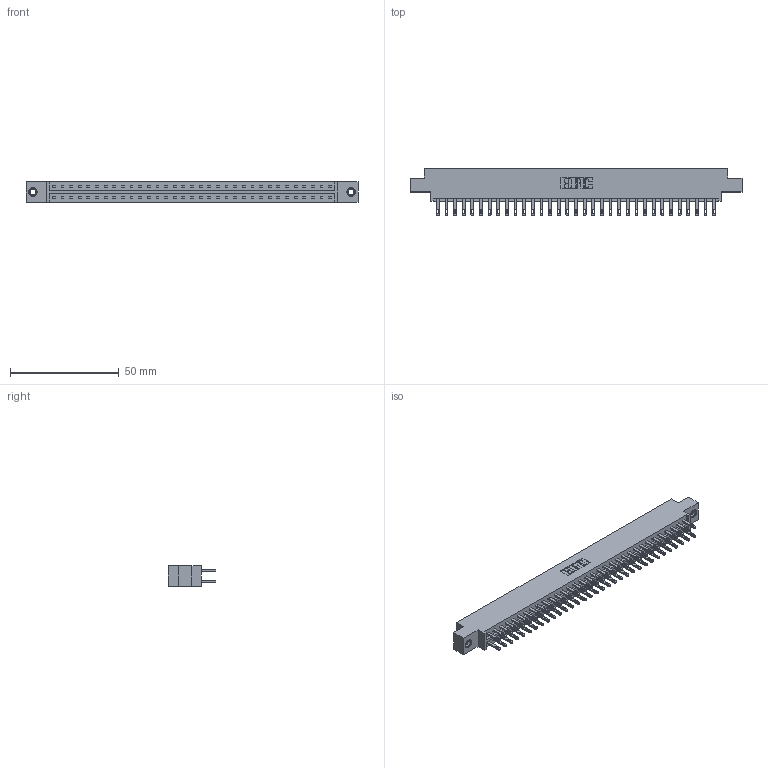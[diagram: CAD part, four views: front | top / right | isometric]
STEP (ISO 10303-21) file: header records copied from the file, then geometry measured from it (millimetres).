
FILE_DESCRIPTION (( 'STEP AP203' ), '1' );
FILE_NAME ('333-066-500-807.STEP', '2018-08-04T10:51:30', ( '' ), ( '' ), 'SwSTEP 2.0', 'SolidWorks 2016', '' );
FILE_SCHEMA (( 'CONFIG_CONTROL_DESIGN' ));
Length unit declared in the file: inch
Products named in the file (4): 333 Part_Offset - .156 Dia - TI; 345-292-001_345-293-100; 345-250-001_345-250-005-103; 333-066-500-807
Assembly tree (69 placements, depth 2):
  333-066-500-807
    333 Part_Offset - .156 Dia - TI
    345-292-001_345-293-100  x66
    345-250-001_345-250-005-103  x2
Bounding box: 152.3 x 21.85 x 9.4 mm (x, y, z)
Volume: 15425 mm3; surface area: 19120.7 mm2
Topology: 69 solids, 69 shells, 3346 faces, 10161 edges, 6766 vertices
Faces by surface type: plane 2086, cylinder 1244, cone 12, torus 4
Entity records: 23642 total; most frequent: CARTESIAN_POINT 3913, ORIENTED_EDGE 3842, DIRECTION 3391, EDGE_CURVE 1921, LINE 1769, VECTOR 1769, VERTEX_POINT 1276, AXIS2_PLACEMENT_3D 811
